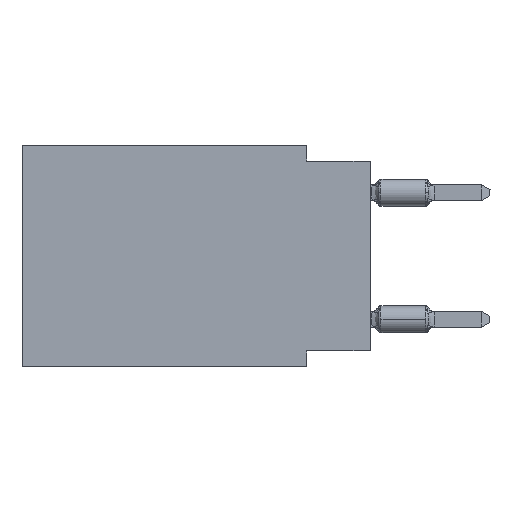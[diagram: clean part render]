
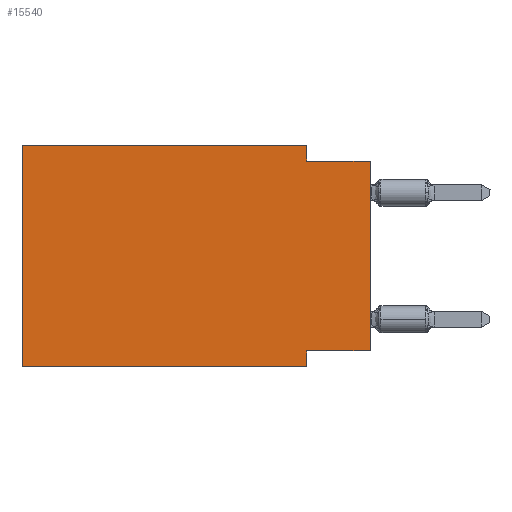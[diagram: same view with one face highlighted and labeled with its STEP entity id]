
A CAD part, left-side view. The second image highlights one B-rep face of the part: STEP entity #15540.
In plain terms, the highlighted planar face has unit normal (-1, 0, 0).
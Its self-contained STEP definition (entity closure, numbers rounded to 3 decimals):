
#628 = LINE ( 'NONE', #12200, #1197 ) ;
#746 = ORIENTED_EDGE ( 'NONE', *, *, #3252, .F. ) ;
#992 = FACE_OUTER_BOUND ( 'NONE', #3918, .T. ) ;
#1197 = VECTOR ( 'NONE', #6287, 1000. ) ;
#1247 = VECTOR ( 'NONE', #12959, 1000. ) ;
#1618 = CARTESIAN_POINT ( 'NONE',  ( 0., 2.54, 0. ) ) ;
#1734 = CARTESIAN_POINT ( 'NONE',  ( 0., 2.54, -8.89 ) ) ;
#2004 = VERTEX_POINT ( 'NONE', #1618 ) ;
#2384 = DIRECTION ( 'NONE',  ( 0., 0., -1. ) ) ;
#2455 = CARTESIAN_POINT ( 'NONE',  ( 0., 0., 0. ) ) ;
#2886 = DIRECTION ( 'NONE',  ( 0., -1., 0. ) ) ;
#3252 = EDGE_CURVE ( 'NONE', #11881, #7961, #6806, .T. ) ;
#3310 = VERTEX_POINT ( 'NONE', #13269 ) ;
#3594 = DIRECTION ( 'NONE',  ( 1., 0., 0. ) ) ;
#3854 = LINE ( 'NONE', #2455, #17578 ) ;
#3918 = EDGE_LOOP ( 'NONE', ( #9187, #3929, #4202, #14170, #5676, #9008, #746, #14378 ) ) ;
#3929 = ORIENTED_EDGE ( 'NONE', *, *, #13606, .F. ) ;
#4123 = DIRECTION ( 'NONE',  ( 0., 1., 0. ) ) ;
#4202 = ORIENTED_EDGE ( 'NONE', *, *, #11530, .F. ) ;
#4341 = CARTESIAN_POINT ( 'NONE',  ( 0., 2.54, -0.635 ) ) ;
#5412 = DIRECTION ( 'NONE',  ( 0., 0., -1. ) ) ;
#5453 = CARTESIAN_POINT ( 'NONE',  ( 0., 2.54, -8.255 ) ) ;
#5538 = VERTEX_POINT ( 'NONE', #7853 ) ;
#5676 = ORIENTED_EDGE ( 'NONE', *, *, #8069, .F. ) ;
#5830 = CARTESIAN_POINT ( 'NONE',  ( 0., 2.54, 0. ) ) ;
#6131 = LINE ( 'NONE', #7248, #7830 ) ;
#6287 = DIRECTION ( 'NONE',  ( 0., 0., 1. ) ) ;
#6806 = LINE ( 'NONE', #12451, #8650 ) ;
#7248 = CARTESIAN_POINT ( 'NONE',  ( 0., 13.97, 0. ) ) ;
#7830 = VECTOR ( 'NONE', #2886, 1000. ) ;
#7853 = CARTESIAN_POINT ( 'NONE',  ( 0., 13.97, 0. ) ) ;
#7961 = VERTEX_POINT ( 'NONE', #1734 ) ;
#8069 = EDGE_CURVE ( 'NONE', #10856, #5538, #628, .T. ) ;
#8479 = VECTOR ( 'NONE', #4123, 1000. ) ;
#8618 = CARTESIAN_POINT ( 'NONE',  ( 0., 13.97, -8.89 ) ) ;
#8650 = VECTOR ( 'NONE', #5412, 1000. ) ;
#9008 = ORIENTED_EDGE ( 'NONE', *, *, #11403, .T. ) ;
#9187 = ORIENTED_EDGE ( 'NONE', *, *, #9716, .T. ) ;
#9716 = EDGE_CURVE ( 'NONE', #14887, #3310, #3854, .T. ) ;
#10403 = EDGE_CURVE ( 'NONE', #5538, #2004, #6131, .T. ) ;
#10514 = CARTESIAN_POINT ( 'NONE',  ( 0., 0., -0.635 ) ) ;
#10856 = VERTEX_POINT ( 'NONE', #17295 ) ;
#11162 = VECTOR ( 'NONE', #11805, 1000. ) ;
#11403 = EDGE_CURVE ( 'NONE', #10856, #7961, #15317, .T. ) ;
#11479 = LINE ( 'NONE', #5830, #17831 ) ;
#11530 = EDGE_CURVE ( 'NONE', #2004, #15252, #11479, .T. ) ;
#11628 = LINE ( 'NONE', #10514, #11162 ) ;
#11805 = DIRECTION ( 'NONE',  ( 0., -1., 0. ) ) ;
#11881 = VERTEX_POINT ( 'NONE', #5453 ) ;
#12200 = CARTESIAN_POINT ( 'NONE',  ( 0., 13.97, 0. ) ) ;
#12451 = CARTESIAN_POINT ( 'NONE',  ( 0., 2.54, -8.89 ) ) ;
#12959 = DIRECTION ( 'NONE',  ( 0., -1., 0. ) ) ;
#13269 = CARTESIAN_POINT ( 'NONE',  ( 0., 0., -0.635 ) ) ;
#13472 = DIRECTION ( 'NONE',  ( 0., 0., 1. ) ) ;
#13494 = PLANE ( 'NONE',  #17427 ) ;
#13606 = EDGE_CURVE ( 'NONE', #15252, #3310, #11628, .T. ) ;
#14170 = ORIENTED_EDGE ( 'NONE', *, *, #10403, .F. ) ;
#14378 = ORIENTED_EDGE ( 'NONE', *, *, #17310, .F. ) ;
#14887 = VERTEX_POINT ( 'NONE', #15823 ) ;
#15252 = VERTEX_POINT ( 'NONE', #4341 ) ;
#15317 = LINE ( 'NONE', #8618, #1247 ) ;
#15540 = ADVANCED_FACE ( 'NONE', ( #992 ), #13494, .F. ) ;
#15823 = CARTESIAN_POINT ( 'NONE',  ( 0., 0., -8.255 ) ) ;
#16283 = CARTESIAN_POINT ( 'NONE',  ( 0., 13.97, 0. ) ) ;
#16813 = CARTESIAN_POINT ( 'NONE',  ( 0., 0., -8.255 ) ) ;
#17135 = DIRECTION ( 'NONE',  ( 0., 0., -1. ) ) ;
#17295 = CARTESIAN_POINT ( 'NONE',  ( 0., 13.97, -8.89 ) ) ;
#17310 = EDGE_CURVE ( 'NONE', #14887, #11881, #18206, .T. ) ;
#17427 = AXIS2_PLACEMENT_3D ( 'NONE', #16283, #3594, #2384 ) ;
#17578 = VECTOR ( 'NONE', #13472, 1000. ) ;
#17831 = VECTOR ( 'NONE', #17135, 1000. ) ;
#18206 = LINE ( 'NONE', #16813, #8479 ) ;
